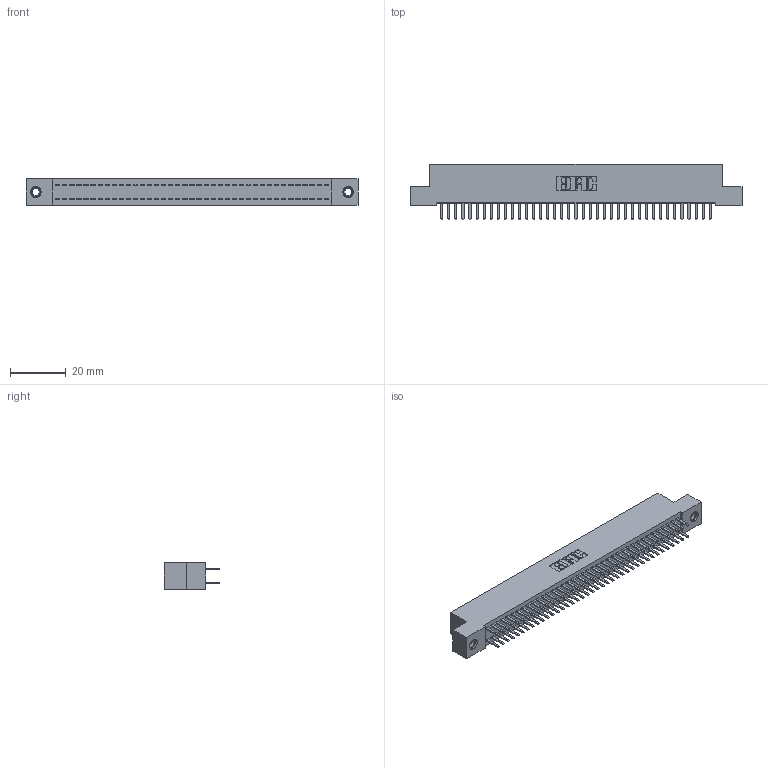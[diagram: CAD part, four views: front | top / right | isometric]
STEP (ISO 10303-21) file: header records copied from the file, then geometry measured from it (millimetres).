
FILE_DESCRIPTION (( 'STEP AP203' ), '1' );
FILE_NAME ('392-078-520-207.STEP', '2018-08-18T01:56:10', ( '' ), ( '' ), 'SwSTEP 2.0', 'SolidWorks 2016', '' );
FILE_SCHEMA (( 'CONFIG_CONTROL_DESIGN' ));
Length unit declared in the file: inch
Products named in the file (4): 342 Part_TI; 345-292-001_345-293-120; 345-250-001_345-250-005-103; 392-078-520-207
Assembly tree (81 placements, depth 2):
  392-078-520-207
    342 Part_TI
    345-292-001_345-293-120  x78
    345-250-001_345-250-005-103  x2
Bounding box: 119.38 x 20.02 x 9.4 mm (x, y, z)
Volume: 10665.1 mm3; surface area: 17231.1 mm2
Topology: 81 solids, 81 shells, 4538 faces, 13149 edges, 8550 vertices
Faces by surface type: plane 3062, cylinder 1460, cone 12, torus 4
Entity records: 26646 total; most frequent: CARTESIAN_POINT 4413, ORIENTED_EDGE 4330, DIRECTION 3795, EDGE_CURVE 2165, VECTOR 2013, LINE 2013, VERTEX_POINT 1436, AXIS2_PLACEMENT_3D 891
